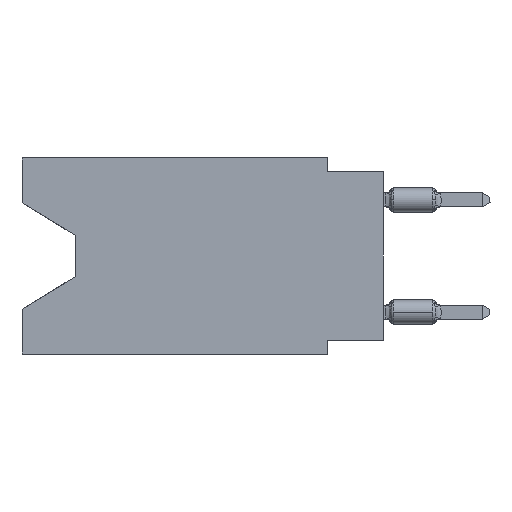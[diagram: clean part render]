
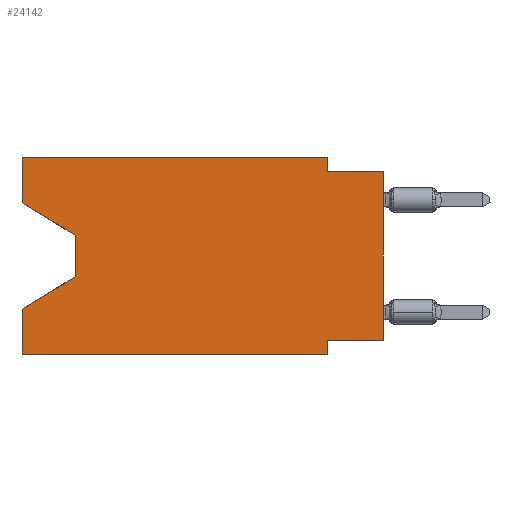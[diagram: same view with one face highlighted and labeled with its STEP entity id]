
A CAD part, left-side view. The second image highlights one B-rep face of the part: STEP entity #24142.
In plain terms, the highlighted planar face has unit normal (-1, 0, 0).
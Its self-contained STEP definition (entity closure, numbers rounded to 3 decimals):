
#1290 = VECTOR ( 'NONE', #49537, 1000. ) ;
#2120 = CARTESIAN_POINT ( 'NONE',  ( 0., 2.54, -0.635 ) ) ;
#2561 = EDGE_CURVE ( 'NONE', #53904, #31447, #51379, .T. ) ;
#2768 = DIRECTION ( 'NONE',  ( 0., 0., 1. ) ) ;
#3445 = CARTESIAN_POINT ( 'NONE',  ( 0., 13.97, -3.505 ) ) ;
#3461 = LINE ( 'NONE', #39077, #31811 ) ;
#4108 = DIRECTION ( 'NONE',  ( 0., 0., -1. ) ) ;
#4110 = ORIENTED_EDGE ( 'NONE', *, *, #25954, .F. ) ;
#4346 = ORIENTED_EDGE ( 'NONE', *, *, #34632, .F. ) ;
#4589 = CARTESIAN_POINT ( 'NONE',  ( 0., 16.383, 0. ) ) ;
#6069 = CARTESIAN_POINT ( 'NONE',  ( 0., 13.97, -5.385 ) ) ;
#6112 = ORIENTED_EDGE ( 'NONE', *, *, #45411, .T. ) ;
#6208 = CARTESIAN_POINT ( 'NONE',  ( 0., 0., -0.635 ) ) ;
#7728 = DIRECTION ( 'NONE',  ( 0., -1., 0. ) ) ;
#7829 = DIRECTION ( 'NONE',  ( 0., 0., 1. ) ) ;
#8806 = EDGE_CURVE ( 'NONE', #14352, #25374, #15614, .T. ) ;
#9515 = VERTEX_POINT ( 'NONE', #38920 ) ;
#9821 = EDGE_CURVE ( 'NONE', #32308, #25374, #12874, .T. ) ;
#10239 = CARTESIAN_POINT ( 'NONE',  ( 0., 16.383, 0. ) ) ;
#10261 = CARTESIAN_POINT ( 'NONE',  ( 0., 2.54, 0. ) ) ;
#10413 = DIRECTION ( 'NONE',  ( 0., -1., 0. ) ) ;
#10535 = ORIENTED_EDGE ( 'NONE', *, *, #2561, .F. ) ;
#10697 = LINE ( 'NONE', #23255, #54583 ) ;
#11207 = EDGE_CURVE ( 'NONE', #15618, #12031, #44654, .T. ) ;
#11354 = VERTEX_POINT ( 'NONE', #41787 ) ;
#11428 = ORIENTED_EDGE ( 'NONE', *, *, #43823, .F. ) ;
#11430 = ORIENTED_EDGE ( 'NONE', *, *, #27125, .T. ) ;
#12031 = VERTEX_POINT ( 'NONE', #45073 ) ;
#12874 = LINE ( 'NONE', #34521, #39637 ) ;
#14352 = VERTEX_POINT ( 'NONE', #27959 ) ;
#15614 = LINE ( 'NONE', #19333, #39405 ) ;
#15618 = VERTEX_POINT ( 'NONE', #19304 ) ;
#16407 = CARTESIAN_POINT ( 'NONE',  ( 0., 16.383, 0. ) ) ;
#16542 = VECTOR ( 'NONE', #19125, 1000. ) ;
#17631 = VERTEX_POINT ( 'NONE', #39708 ) ;
#19083 = EDGE_LOOP ( 'NONE', ( #30740, #33148, #6112, #10535, #11430, #11428, #4110, #39365, #33299, #55817, #4346, #40221 ) ) ;
#19125 = DIRECTION ( 'NONE',  ( 0., 0., -1. ) ) ;
#19304 = CARTESIAN_POINT ( 'NONE',  ( 0., 16.383, -2.038 ) ) ;
#19333 = CARTESIAN_POINT ( 'NONE',  ( 0., 0., 0. ) ) ;
#19958 = DIRECTION ( 'NONE',  ( 1., 0., 0. ) ) ;
#22549 = LINE ( 'NONE', #10261, #16542 ) ;
#23255 = CARTESIAN_POINT ( 'NONE',  ( 0., 16.383, -8.89 ) ) ;
#23880 = CARTESIAN_POINT ( 'NONE',  ( 0., 16.383, -2.038 ) ) ;
#24142 = ADVANCED_FACE ( 'NONE', ( #41585 ), #29062, .F. ) ;
#25147 = DIRECTION ( 'NONE',  ( 0., 0.855, -0.519 ) ) ;
#25374 = VERTEX_POINT ( 'NONE', #6208 ) ;
#25893 = VECTOR ( 'NONE', #25147, 1000. ) ;
#25954 = EDGE_CURVE ( 'NONE', #14352, #51085, #3461, .T. ) ;
#27125 = EDGE_CURVE ( 'NONE', #53904, #50254, #10697, .T. ) ;
#27126 = VECTOR ( 'NONE', #41224, 1000. ) ;
#27650 = LINE ( 'NONE', #10239, #1290 ) ;
#27959 = CARTESIAN_POINT ( 'NONE',  ( 0., 0., -8.255 ) ) ;
#29062 = PLANE ( 'NONE',  #51599 ) ;
#30740 = ORIENTED_EDGE ( 'NONE', *, *, #11207, .T. ) ;
#30866 = VECTOR ( 'NONE', #7829, 1000. ) ;
#31447 = VERTEX_POINT ( 'NONE', #54370 ) ;
#31811 = VECTOR ( 'NONE', #47035, 1000. ) ;
#32308 = VERTEX_POINT ( 'NONE', #2120 ) ;
#33148 = ORIENTED_EDGE ( 'NONE', *, *, #50938, .T. ) ;
#33299 = ORIENTED_EDGE ( 'NONE', *, *, #9821, .F. ) ;
#33654 = DIRECTION ( 'NONE',  ( 0., -1., 0. ) ) ;
#34521 = CARTESIAN_POINT ( 'NONE',  ( 0., 0., -0.635 ) ) ;
#34632 = EDGE_CURVE ( 'NONE', #17631, #9515, #47312, .T. ) ;
#35834 = EDGE_CURVE ( 'NONE', #9515, #32308, #22549, .T. ) ;
#38576 = LINE ( 'NONE', #43137, #48789 ) ;
#38920 = CARTESIAN_POINT ( 'NONE',  ( 0., 2.54, 0. ) ) ;
#39077 = CARTESIAN_POINT ( 'NONE',  ( 0., 0., -8.255 ) ) ;
#39365 = ORIENTED_EDGE ( 'NONE', *, *, #8806, .T. ) ;
#39405 = VECTOR ( 'NONE', #2768, 1000. ) ;
#39637 = VECTOR ( 'NONE', #7728, 1000. ) ;
#39708 = CARTESIAN_POINT ( 'NONE',  ( 0., 16.383, 0. ) ) ;
#40221 = ORIENTED_EDGE ( 'NONE', *, *, #40581, .F. ) ;
#40581 = EDGE_CURVE ( 'NONE', #15618, #17631, #27650, .T. ) ;
#41224 = DIRECTION ( 'NONE',  ( 0., -0.855, -0.519 ) ) ;
#41348 = VECTOR ( 'NONE', #33654, 1000. ) ;
#41585 = FACE_OUTER_BOUND ( 'NONE', #19083, .T. ) ;
#41787 = CARTESIAN_POINT ( 'NONE',  ( 0., 13.97, -5.385 ) ) ;
#43137 = CARTESIAN_POINT ( 'NONE',  ( 0., 2.54, -8.89 ) ) ;
#43823 = EDGE_CURVE ( 'NONE', #51085, #50254, #38576, .T. ) ;
#44176 = CARTESIAN_POINT ( 'NONE',  ( 0., 2.54, -8.255 ) ) ;
#44654 = LINE ( 'NONE', #23880, #27126 ) ;
#44772 = CARTESIAN_POINT ( 'NONE',  ( 0., 16.383, -8.89 ) ) ;
#45073 = CARTESIAN_POINT ( 'NONE',  ( 0., 13.97, -3.505 ) ) ;
#45092 = LINE ( 'NONE', #6069, #25893 ) ;
#45411 = EDGE_CURVE ( 'NONE', #11354, #31447, #45092, .T. ) ;
#45545 = VECTOR ( 'NONE', #51272, 1000. ) ;
#46955 = CARTESIAN_POINT ( 'NONE',  ( 0., 16.383, 0. ) ) ;
#47035 = DIRECTION ( 'NONE',  ( 0., 1., 0. ) ) ;
#47312 = LINE ( 'NONE', #4589, #41348 ) ;
#47587 = LINE ( 'NONE', #3445, #45545 ) ;
#48789 = VECTOR ( 'NONE', #4108, 1000. ) ;
#49537 = DIRECTION ( 'NONE',  ( 0., 0., 1. ) ) ;
#50254 = VERTEX_POINT ( 'NONE', #53933 ) ;
#50640 = DIRECTION ( 'NONE',  ( 0., 0., -1. ) ) ;
#50938 = EDGE_CURVE ( 'NONE', #12031, #11354, #47587, .T. ) ;
#51085 = VERTEX_POINT ( 'NONE', #44176 ) ;
#51272 = DIRECTION ( 'NONE',  ( 0., 0., -1. ) ) ;
#51379 = LINE ( 'NONE', #16407, #30866 ) ;
#51599 = AXIS2_PLACEMENT_3D ( 'NONE', #46955, #19958, #50640 ) ;
#53904 = VERTEX_POINT ( 'NONE', #44772 ) ;
#53933 = CARTESIAN_POINT ( 'NONE',  ( 0., 2.54, -8.89 ) ) ;
#54370 = CARTESIAN_POINT ( 'NONE',  ( 0., 16.383, -6.852 ) ) ;
#54583 = VECTOR ( 'NONE', #10413, 1000. ) ;
#55817 = ORIENTED_EDGE ( 'NONE', *, *, #35834, .F. ) ;
